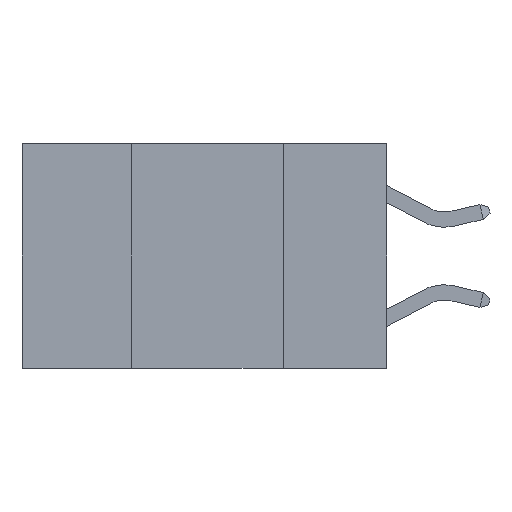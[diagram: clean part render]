
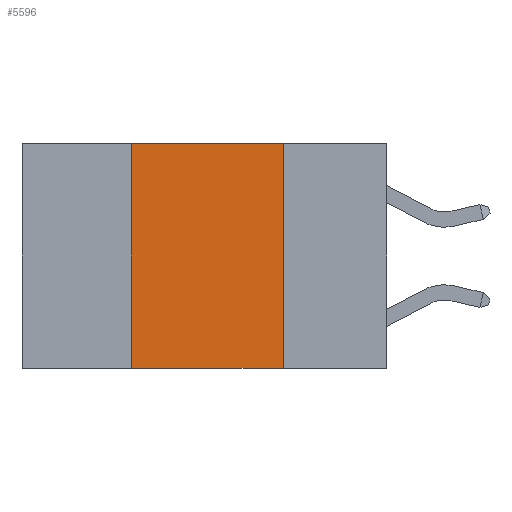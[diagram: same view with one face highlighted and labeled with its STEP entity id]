
A CAD part, left-side view. The second image highlights one B-rep face of the part: STEP entity #5596.
In plain terms, the highlighted planar face has unit normal (-1, 0, 0).
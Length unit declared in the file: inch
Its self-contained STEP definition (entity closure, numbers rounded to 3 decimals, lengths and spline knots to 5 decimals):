
#822 = DIRECTION ( 'NONE',  ( 1., 0., 0. ) ) ;
#1104 = DIRECTION ( 'NONE',  ( 0., -1., 0. ) ) ;
#1164 = EDGE_CURVE ( 'NONE', #5732, #5078, #5826, .T. ) ;
#1236 = CARTESIAN_POINT ( 'NONE',  ( 0., 0.6, 0. ) ) ;
#1989 = VECTOR ( 'NONE', #1104, 39.37008 ) ;
#2006 = CARTESIAN_POINT ( 'NONE',  ( 0., 0.17, 0. ) ) ;
#2534 = ORIENTED_EDGE ( 'NONE', *, *, #8082, .F. ) ;
#2790 = VERTEX_POINT ( 'NONE', #2006 ) ;
#3291 = CARTESIAN_POINT ( 'NONE',  ( 0., 0.42, 0. ) ) ;
#4014 = DIRECTION ( 'NONE',  ( 0., 0., 1. ) ) ;
#4290 = DIRECTION ( 'NONE',  ( 0., -1., 0. ) ) ;
#4697 = CARTESIAN_POINT ( 'NONE',  ( 0., 0.17, -0.37 ) ) ;
#4814 = PLANE ( 'NONE',  #7906 ) ;
#4872 = LINE ( 'NONE', #7152, #1989 ) ;
#5078 = VERTEX_POINT ( 'NONE', #7414 ) ;
#5381 = ORIENTED_EDGE ( 'NONE', *, *, #8813, .T. ) ;
#5436 = DIRECTION ( 'NONE',  ( 0., 0., -1. ) ) ;
#5485 = CARTESIAN_POINT ( 'NONE',  ( 0., 0.6, 0. ) ) ;
#5490 = VERTEX_POINT ( 'NONE', #4697 ) ;
#5596 = ADVANCED_FACE ( 'NONE', ( #7712 ), #4814, .F. ) ;
#5732 = VERTEX_POINT ( 'NONE', #8717 ) ;
#5817 = LINE ( 'NONE', #1236, #6154 ) ;
#5826 = LINE ( 'NONE', #3291, #5980 ) ;
#5980 = VECTOR ( 'NONE', #4014, 39.37008 ) ;
#6154 = VECTOR ( 'NONE', #4290, 39.37008 ) ;
#6176 = DIRECTION ( 'NONE',  ( 0., 0., -1. ) ) ;
#7074 = ORIENTED_EDGE ( 'NONE', *, *, #1164, .F. ) ;
#7152 = CARTESIAN_POINT ( 'NONE',  ( 0., 0.6, -0.37 ) ) ;
#7414 = CARTESIAN_POINT ( 'NONE',  ( 0., 0.42, 0. ) ) ;
#7621 = LINE ( 'NONE', #8518, #9756 ) ;
#7712 = FACE_OUTER_BOUND ( 'NONE', #8418, .T. ) ;
#7906 = AXIS2_PLACEMENT_3D ( 'NONE', #5485, #822, #5436 ) ;
#8082 = EDGE_CURVE ( 'NONE', #5078, #2790, #5817, .T. ) ;
#8418 = EDGE_LOOP ( 'NONE', ( #9377, #2534, #7074, #5381 ) ) ;
#8518 = CARTESIAN_POINT ( 'NONE',  ( 0., 0.17, 0. ) ) ;
#8612 = EDGE_CURVE ( 'NONE', #2790, #5490, #7621, .T. ) ;
#8717 = CARTESIAN_POINT ( 'NONE',  ( 0., 0.42, -0.37 ) ) ;
#8813 = EDGE_CURVE ( 'NONE', #5732, #5490, #4872, .T. ) ;
#9377 = ORIENTED_EDGE ( 'NONE', *, *, #8612, .F. ) ;
#9756 = VECTOR ( 'NONE', #6176, 39.37008 ) ;
